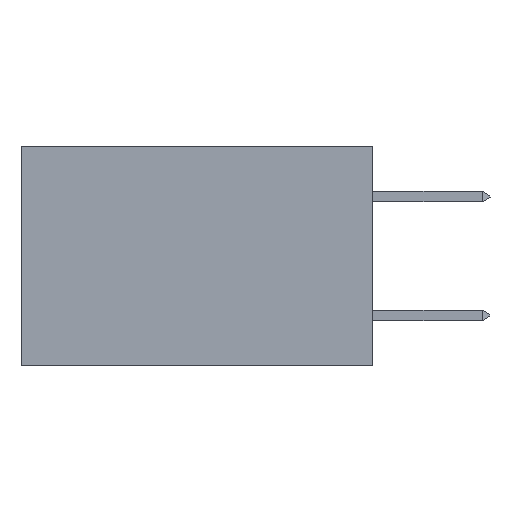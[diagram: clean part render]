
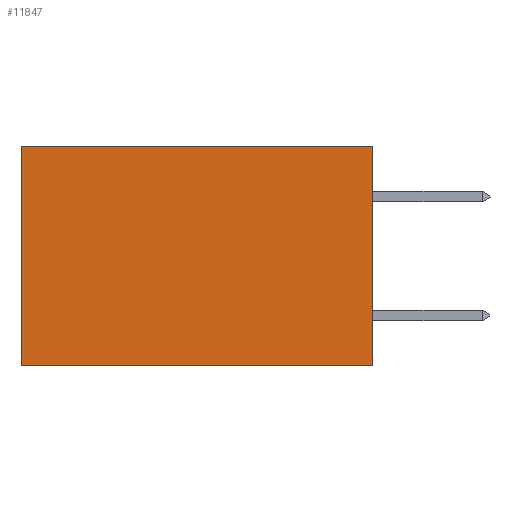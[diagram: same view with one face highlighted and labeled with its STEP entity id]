
A CAD part, left-side view. The second image highlights one B-rep face of the part: STEP entity #11847.
In plain terms, the highlighted planar face has unit normal (-1, 0, 0).
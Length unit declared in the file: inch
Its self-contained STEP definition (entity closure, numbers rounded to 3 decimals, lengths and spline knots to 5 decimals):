
#321 = PLANE ( 'NONE',  #15186 ) ;
#915 = EDGE_LOOP ( 'NONE', ( #14848, #8674, #8512, #1106 ) ) ;
#1106 = ORIENTED_EDGE ( 'NONE', *, *, #11752, .T. ) ;
#1277 = CARTESIAN_POINT ( 'NONE',  ( 0.277, 0., -0.37 ) ) ;
#2024 = EDGE_CURVE ( 'NONE', #8969, #10718, #6434, .T. ) ;
#3040 = VECTOR ( 'NONE', #4097, 39.37008 ) ;
#3535 = EDGE_CURVE ( 'NONE', #10007, #10718, #4788, .T. ) ;
#4097 = DIRECTION ( 'NONE',  ( 0., 1., 0. ) ) ;
#4236 = CARTESIAN_POINT ( 'NONE',  ( 0.277, 0., -0.37 ) ) ;
#4788 = LINE ( 'NONE', #7536, #16067 ) ;
#5338 = DIRECTION ( 'NONE',  ( 0., 1., 0. ) ) ;
#5432 = CARTESIAN_POINT ( 'NONE',  ( 0.277, 0., -0.37 ) ) ;
#5503 = DIRECTION ( 'NONE',  ( 0., 0., -1. ) ) ;
#5578 = VECTOR ( 'NONE', #13852, 39.37008 ) ;
#6305 = CARTESIAN_POINT ( 'NONE',  ( 0.277, 0., -0.37 ) ) ;
#6434 = LINE ( 'NONE', #5432, #3040 ) ;
#7499 = DIRECTION ( 'NONE',  ( 0., 0., -1. ) ) ;
#7536 = CARTESIAN_POINT ( 'NONE',  ( 0.277, 0.59, -0.37 ) ) ;
#8088 = FACE_OUTER_BOUND ( 'NONE', #915, .T. ) ;
#8225 = EDGE_CURVE ( 'NONE', #14803, #8969, #9010, .T. ) ;
#8512 = ORIENTED_EDGE ( 'NONE', *, *, #8225, .F. ) ;
#8674 = ORIENTED_EDGE ( 'NONE', *, *, #2024, .F. ) ;
#8969 = VERTEX_POINT ( 'NONE', #1277 ) ;
#9010 = LINE ( 'NONE', #6305, #5578 ) ;
#9707 = VECTOR ( 'NONE', #5338, 39.37008 ) ;
#10007 = VERTEX_POINT ( 'NONE', #15954 ) ;
#10718 = VERTEX_POINT ( 'NONE', #12308 ) ;
#11752 = EDGE_CURVE ( 'NONE', #14803, #10007, #16331, .T. ) ;
#11847 = ADVANCED_FACE ( 'NONE', ( #8088 ), #321, .F. ) ;
#12308 = CARTESIAN_POINT ( 'NONE',  ( 0.277, 0.59, -0.37 ) ) ;
#12949 = CARTESIAN_POINT ( 'NONE',  ( 0.277, 0., 0. ) ) ;
#13085 = DIRECTION ( 'NONE',  ( 1., 0., 0. ) ) ;
#13346 = CARTESIAN_POINT ( 'NONE',  ( 0.277, 0., 0. ) ) ;
#13852 = DIRECTION ( 'NONE',  ( 0., 0., -1. ) ) ;
#14803 = VERTEX_POINT ( 'NONE', #13346 ) ;
#14848 = ORIENTED_EDGE ( 'NONE', *, *, #3535, .T. ) ;
#15186 = AXIS2_PLACEMENT_3D ( 'NONE', #4236, #13085, #5503 ) ;
#15954 = CARTESIAN_POINT ( 'NONE',  ( 0.277, 0.59, 0. ) ) ;
#16067 = VECTOR ( 'NONE', #7499, 39.37008 ) ;
#16331 = LINE ( 'NONE', #12949, #9707 ) ;
